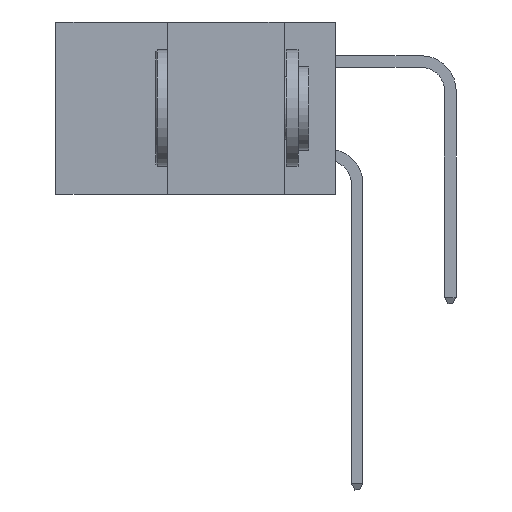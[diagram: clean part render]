
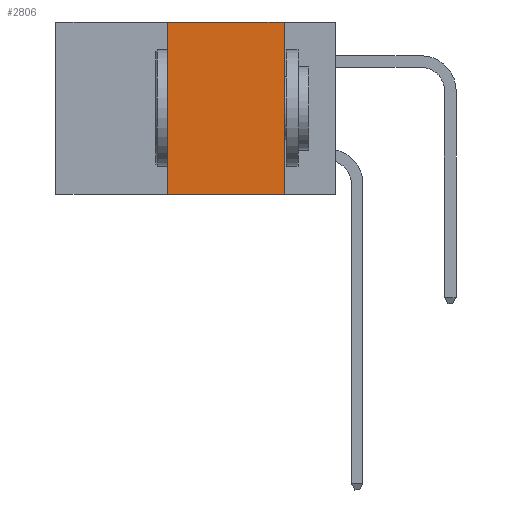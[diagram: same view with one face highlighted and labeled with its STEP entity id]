
A CAD part, left-side view. The second image highlights one B-rep face of the part: STEP entity #2806.
In plain terms, the highlighted planar face has unit normal (-1, 0, 0).
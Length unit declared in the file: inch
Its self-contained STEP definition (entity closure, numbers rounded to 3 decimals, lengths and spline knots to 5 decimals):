
#122 = ORIENTED_EDGE ( 'NONE', *, *, #10621, .F. ) ;
#127 = EDGE_LOOP ( 'NONE', ( #122, #4371, #5490, #307 ) ) ;
#307 = ORIENTED_EDGE ( 'NONE', *, *, #2288, .T. ) ;
#783 = LINE ( 'NONE', #13502, #2813 ) ;
#1530 = VERTEX_POINT ( 'NONE', #5341 ) ;
#1710 = FACE_OUTER_BOUND ( 'NONE', #127, .T. ) ;
#2288 = EDGE_CURVE ( 'NONE', #1530, #9380, #15006, .T. ) ;
#2806 = ADVANCED_FACE ( 'NONE', ( #1710 ), #7297, .F. ) ;
#2813 = VECTOR ( 'NONE', #6416, 39.37008 ) ;
#3119 = DIRECTION ( 'NONE',  ( 0., -1., 0. ) ) ;
#4371 = ORIENTED_EDGE ( 'NONE', *, *, #11533, .F. ) ;
#4992 = CARTESIAN_POINT ( 'NONE',  ( 0., 0.11, 0. ) ) ;
#5126 = LINE ( 'NONE', #12593, #5500 ) ;
#5196 = CARTESIAN_POINT ( 'NONE',  ( 0., 0.11, -0.37 ) ) ;
#5341 = CARTESIAN_POINT ( 'NONE',  ( 0., 0.36, -0.37 ) ) ;
#5490 = ORIENTED_EDGE ( 'NONE', *, *, #15059, .F. ) ;
#5500 = VECTOR ( 'NONE', #9021, 39.37008 ) ;
#5651 = CARTESIAN_POINT ( 'NONE',  ( 0., 0.6, -0.37 ) ) ;
#6242 = AXIS2_PLACEMENT_3D ( 'NONE', #6486, #7477, #6571 ) ;
#6416 = DIRECTION ( 'NONE',  ( 0., -1., 0. ) ) ;
#6486 = CARTESIAN_POINT ( 'NONE',  ( 0., 0.6, 0. ) ) ;
#6571 = DIRECTION ( 'NONE',  ( 0., 0., -1. ) ) ;
#7297 = PLANE ( 'NONE',  #6242 ) ;
#7477 = DIRECTION ( 'NONE',  ( 1., 0., 0. ) ) ;
#8388 = VECTOR ( 'NONE', #3119, 39.37008 ) ;
#9021 = DIRECTION ( 'NONE',  ( 0., 0., 1. ) ) ;
#9380 = VERTEX_POINT ( 'NONE', #5196 ) ;
#9681 = CARTESIAN_POINT ( 'NONE',  ( 0., 0.36, 0. ) ) ;
#9918 = VERTEX_POINT ( 'NONE', #9681 ) ;
#10621 = EDGE_CURVE ( 'NONE', #10756, #9380, #11563, .T. ) ;
#10756 = VERTEX_POINT ( 'NONE', #4992 ) ;
#11533 = EDGE_CURVE ( 'NONE', #9918, #10756, #783, .T. ) ;
#11563 = LINE ( 'NONE', #13024, #14308 ) ;
#12593 = CARTESIAN_POINT ( 'NONE',  ( 0., 0.36, 0. ) ) ;
#13024 = CARTESIAN_POINT ( 'NONE',  ( 0., 0.11, 0. ) ) ;
#13502 = CARTESIAN_POINT ( 'NONE',  ( 0., 0.6, 0. ) ) ;
#14187 = DIRECTION ( 'NONE',  ( 0., 0., -1. ) ) ;
#14308 = VECTOR ( 'NONE', #14187, 39.37008 ) ;
#15006 = LINE ( 'NONE', #5651, #8388 ) ;
#15059 = EDGE_CURVE ( 'NONE', #1530, #9918, #5126, .T. ) ;
